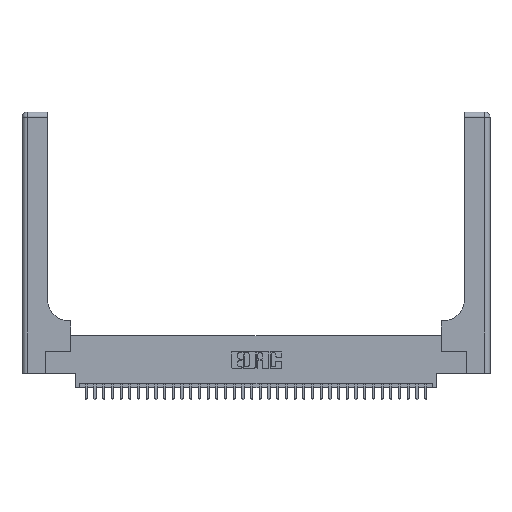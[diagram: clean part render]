
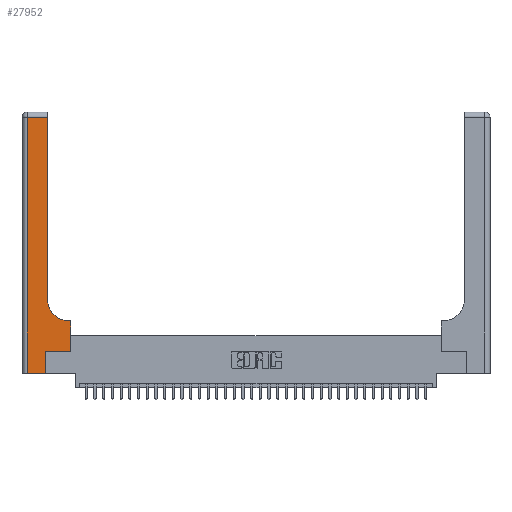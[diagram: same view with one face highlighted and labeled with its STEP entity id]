
A CAD part, top view. The second image highlights one B-rep face of the part: STEP entity #27952.
In plain terms, the highlighted planar face has unit normal (0, 0, 1).
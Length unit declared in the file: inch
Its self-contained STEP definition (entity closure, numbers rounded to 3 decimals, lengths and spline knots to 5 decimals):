
#63 = CARTESIAN_POINT ( 'NONE',  ( 0.06, 3., 0.37 ) ) ;
#185 = DIRECTION ( 'NONE',  ( 0., -1., 0. ) ) ;
#331 = LINE ( 'NONE', #14490, #22300 ) ;
#1202 = VERTEX_POINT ( 'NONE', #3144 ) ;
#1245 = AXIS2_PLACEMENT_3D ( 'NONE', #20619, #3499, #23517 ) ;
#1379 = DIRECTION ( 'NONE',  ( -1., 0., 0. ) ) ;
#1844 = EDGE_CURVE ( 'NONE', #5004, #3908, #11754, .T. ) ;
#2716 = CARTESIAN_POINT ( 'NONE',  ( 0.269, 0.25, 0.37 ) ) ;
#2880 = ORIENTED_EDGE ( 'NONE', *, *, #6350, .T. ) ;
#3144 = CARTESIAN_POINT ( 'NONE',  ( 0.2915, 2.94, 0.37 ) ) ;
#3406 = ORIENTED_EDGE ( 'NONE', *, *, #13354, .T. ) ;
#3499 = DIRECTION ( 'NONE',  ( 0., 0., -1. ) ) ;
#3908 = VERTEX_POINT ( 'NONE', #21180 ) ;
#4160 = VECTOR ( 'NONE', #185, 39.37008 ) ;
#5004 = VERTEX_POINT ( 'NONE', #6483 ) ;
#5339 = EDGE_CURVE ( 'NONE', #19255, #11721, #5788, .T. ) ;
#5788 = LINE ( 'NONE', #2716, #35226 ) ;
#6350 = EDGE_CURVE ( 'NONE', #33547, #19255, #32979, .T. ) ;
#6483 = CARTESIAN_POINT ( 'NONE',  ( 0.06, 2.94, 0.37 ) ) ;
#8070 = ORIENTED_EDGE ( 'NONE', *, *, #1844, .T. ) ;
#8964 = CARTESIAN_POINT ( 'NONE',  ( 0., 0., 0.37 ) ) ;
#9763 = PLANE ( 'NONE',  #18489 ) ;
#9919 = LINE ( 'NONE', #8964, #24277 ) ;
#10775 = CARTESIAN_POINT ( 'NONE',  ( 0.269, 0., 0.37 ) ) ;
#11094 = EDGE_CURVE ( 'NONE', #3908, #33547, #9919, .T. ) ;
#11436 = ORIENTED_EDGE ( 'NONE', *, *, #5339, .T. ) ;
#11441 = LINE ( 'NONE', #23339, #33323 ) ;
#11721 = VERTEX_POINT ( 'NONE', #15598 ) ;
#11754 = LINE ( 'NONE', #63, #4160 ) ;
#13354 = EDGE_CURVE ( 'NONE', #1202, #5004, #331, .T. ) ;
#13396 = VERTEX_POINT ( 'NONE', #20361 ) ;
#13631 = CARTESIAN_POINT ( 'NONE',  ( 0.5415, 0.6, 0.37 ) ) ;
#13645 = FACE_OUTER_BOUND ( 'NONE', #16008, .T. ) ;
#13747 = VERTEX_POINT ( 'NONE', #21735 ) ;
#14221 = DIRECTION ( 'NONE',  ( 1., 0., 0. ) ) ;
#14490 = CARTESIAN_POINT ( 'NONE',  ( 0., 2.94, 0.37 ) ) ;
#14776 = EDGE_CURVE ( 'NONE', #35045, #13747, #29758, .T. ) ;
#15053 = EDGE_CURVE ( 'NONE', #11721, #13396, #20809, .T. ) ;
#15538 = DIRECTION ( 'NONE',  ( -1., 0., 0. ) ) ;
#15598 = CARTESIAN_POINT ( 'NONE',  ( 0.5585, 0.25, 0.37 ) ) ;
#16008 = EDGE_LOOP ( 'NONE', ( #16747, #3406, #8070, #17391, #2880, #11436, #19943, #32922, #32985 ) ) ;
#16747 = ORIENTED_EDGE ( 'NONE', *, *, #27291, .T. ) ;
#17391 = ORIENTED_EDGE ( 'NONE', *, *, #11094, .T. ) ;
#18290 = LINE ( 'NONE', #24180, #25055 ) ;
#18339 = CARTESIAN_POINT ( 'NONE',  ( 0.269, 0., 0.37 ) ) ;
#18489 = AXIS2_PLACEMENT_3D ( 'NONE', #29756, #32594, #15538 ) ;
#18866 = DIRECTION ( 'NONE',  ( 0., 1., 0. ) ) ;
#19255 = VERTEX_POINT ( 'NONE', #28075 ) ;
#19943 = ORIENTED_EDGE ( 'NONE', *, *, #15053, .T. ) ;
#20361 = CARTESIAN_POINT ( 'NONE',  ( 0.5585, 0.6, 0.37 ) ) ;
#20619 = CARTESIAN_POINT ( 'NONE',  ( 0.5415, 0.85, 0.37 ) ) ;
#20809 = LINE ( 'NONE', #33062, #28409 ) ;
#21180 = CARTESIAN_POINT ( 'NONE',  ( 0.06, 0., 0.37 ) ) ;
#21735 = CARTESIAN_POINT ( 'NONE',  ( 0.2915, 0.85, 0.37 ) ) ;
#22300 = VECTOR ( 'NONE', #25984, 39.37008 ) ;
#22435 = DIRECTION ( 'NONE',  ( 0., 1., 0. ) ) ;
#23339 = CARTESIAN_POINT ( 'NONE',  ( 0.2915, 3., 0.37 ) ) ;
#23517 = DIRECTION ( 'NONE',  ( 1., 0., 0. ) ) ;
#24180 = CARTESIAN_POINT ( 'NONE',  ( 0.2915, 0.6, 0.37 ) ) ;
#24277 = VECTOR ( 'NONE', #31681, 39.37008 ) ;
#25055 = VECTOR ( 'NONE', #1379, 39.37008 ) ;
#25984 = DIRECTION ( 'NONE',  ( -1., 0., 0. ) ) ;
#26192 = DIRECTION ( 'NONE',  ( 0., 1., 0. ) ) ;
#27291 = EDGE_CURVE ( 'NONE', #13747, #1202, #11441, .T. ) ;
#27952 = ADVANCED_FACE ( 'NONE', ( #13645 ), #9763, .F. ) ;
#28075 = CARTESIAN_POINT ( 'NONE',  ( 0.269, 0.25, 0.37 ) ) ;
#28409 = VECTOR ( 'NONE', #18866, 39.37008 ) ;
#29756 = CARTESIAN_POINT ( 'NONE',  ( 0., 3., 0.37 ) ) ;
#29758 = CIRCLE ( 'NONE', #1245, 0.25 ) ;
#31681 = DIRECTION ( 'NONE',  ( 1., 0., 0. ) ) ;
#32064 = VECTOR ( 'NONE', #22435, 39.37008 ) ;
#32594 = DIRECTION ( 'NONE',  ( 0., 0., -1. ) ) ;
#32922 = ORIENTED_EDGE ( 'NONE', *, *, #36094, .T. ) ;
#32979 = LINE ( 'NONE', #10775, #32064 ) ;
#32985 = ORIENTED_EDGE ( 'NONE', *, *, #14776, .T. ) ;
#33062 = CARTESIAN_POINT ( 'NONE',  ( 0.5585, 0.25, 0.37 ) ) ;
#33323 = VECTOR ( 'NONE', #26192, 39.37008 ) ;
#33547 = VERTEX_POINT ( 'NONE', #18339 ) ;
#35045 = VERTEX_POINT ( 'NONE', #13631 ) ;
#35226 = VECTOR ( 'NONE', #14221, 39.37008 ) ;
#36094 = EDGE_CURVE ( 'NONE', #13396, #35045, #18290, .T. ) ;
